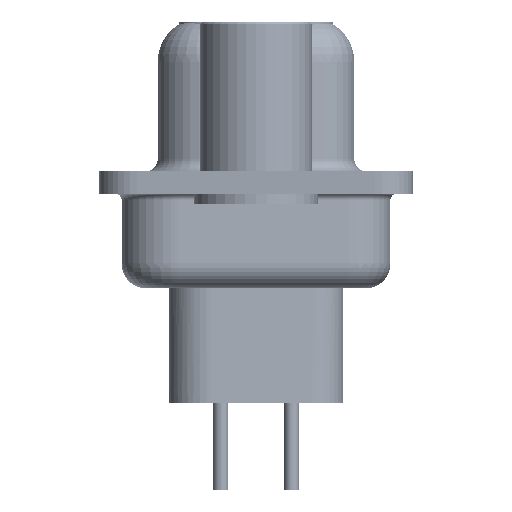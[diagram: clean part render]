
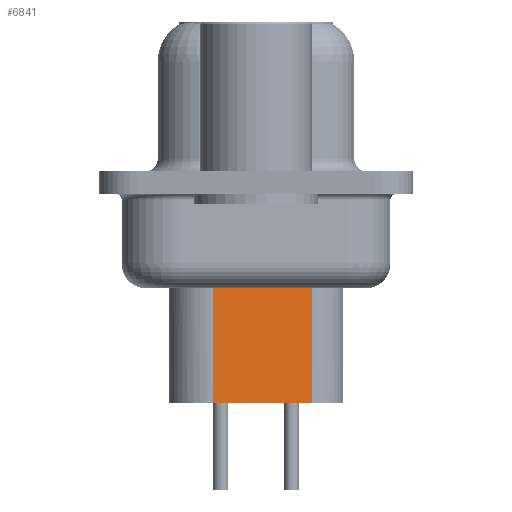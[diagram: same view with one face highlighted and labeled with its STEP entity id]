
A CAD part, left-side view. The second image highlights one B-rep face of the part: STEP entity #6841.
In plain terms, the highlighted planar face has unit normal (-0.985, -0.174, 0).
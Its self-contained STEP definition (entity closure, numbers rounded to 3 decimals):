
#1286 = CARTESIAN_POINT ( 'NONE',  ( 4.353, 2.709, -3.975 ) ) ;
#1542 = ORIENTED_EDGE ( 'NONE', *, *, #16829, .T. ) ;
#1986 = CARTESIAN_POINT ( 'NONE',  ( 4.524, 1.74, -8.85 ) ) ;
#3500 = DIRECTION ( 'NONE',  ( -0.174, 0.985, 0. ) ) ;
#6841 = ADVANCED_FACE ( 'NONE', ( #27625 ), #14736, .T. ) ;
#8922 = DIRECTION ( 'NONE',  ( 0.174, -0.985, 0. ) ) ;
#9668 = ORIENTED_EDGE ( 'NONE', *, *, #10929, .T. ) ;
#9715 = CARTESIAN_POINT ( 'NONE',  ( 4.524, 1.74, -8.85 ) ) ;
#9933 = VECTOR ( 'NONE', #3500, 1000. ) ;
#9979 = EDGE_LOOP ( 'NONE', ( #20969, #1542, #9668, #22960 ) ) ;
#10851 = DIRECTION ( 'NONE',  ( 0., 0., -1. ) ) ;
#10929 = EDGE_CURVE ( 'NONE', #20521, #28361, #29186, .T. ) ;
#12206 = LINE ( 'NONE', #30003, #14662 ) ;
#13412 = CARTESIAN_POINT ( 'NONE',  ( 4.524, 1.74, -3.1 ) ) ;
#14060 = DIRECTION ( 'NONE',  ( -0.985, -0.174, 0. ) ) ;
#14303 = CARTESIAN_POINT ( 'NONE',  ( 4.524, 1.74, -3.975 ) ) ;
#14662 = VECTOR ( 'NONE', #24929, 1000. ) ;
#14736 = PLANE ( 'NONE',  #33405 ) ;
#15073 = VERTEX_POINT ( 'NONE', #25199 ) ;
#15323 = LINE ( 'NONE', #1986, #25578 ) ;
#16496 = LINE ( 'NONE', #1286, #9933 ) ;
#16829 = EDGE_CURVE ( 'NONE', #33528, #20521, #16496, .T. ) ;
#17872 = VECTOR ( 'NONE', #10851, 1000. ) ;
#20521 = VERTEX_POINT ( 'NONE', #14303 ) ;
#20969 = ORIENTED_EDGE ( 'NONE', *, *, #26287, .F. ) ;
#22960 = ORIENTED_EDGE ( 'NONE', *, *, #31118, .F. ) ;
#24929 = DIRECTION ( 'NONE',  ( 0., 0., -1. ) ) ;
#25079 = CARTESIAN_POINT ( 'NONE',  ( 4.524, 1.74, -3.1 ) ) ;
#25199 = CARTESIAN_POINT ( 'NONE',  ( 5.229, -2.26, -8.85 ) ) ;
#25578 = VECTOR ( 'NONE', #33122, 1000. ) ;
#26287 = EDGE_CURVE ( 'NONE', #33528, #15073, #12206, .T. ) ;
#27625 = FACE_OUTER_BOUND ( 'NONE', #9979, .T. ) ;
#28361 = VERTEX_POINT ( 'NONE', #9715 ) ;
#29186 = LINE ( 'NONE', #13412, #17872 ) ;
#30003 = CARTESIAN_POINT ( 'NONE',  ( 5.229, -2.26, -3.1 ) ) ;
#31118 = EDGE_CURVE ( 'NONE', #15073, #28361, #15323, .T. ) ;
#32752 = CARTESIAN_POINT ( 'NONE',  ( 5.229, -2.26, -3.975 ) ) ;
#33122 = DIRECTION ( 'NONE',  ( -0.174, 0.985, 0. ) ) ;
#33405 = AXIS2_PLACEMENT_3D ( 'NONE', #25079, #14060, #8922 ) ;
#33528 = VERTEX_POINT ( 'NONE', #32752 ) ;
